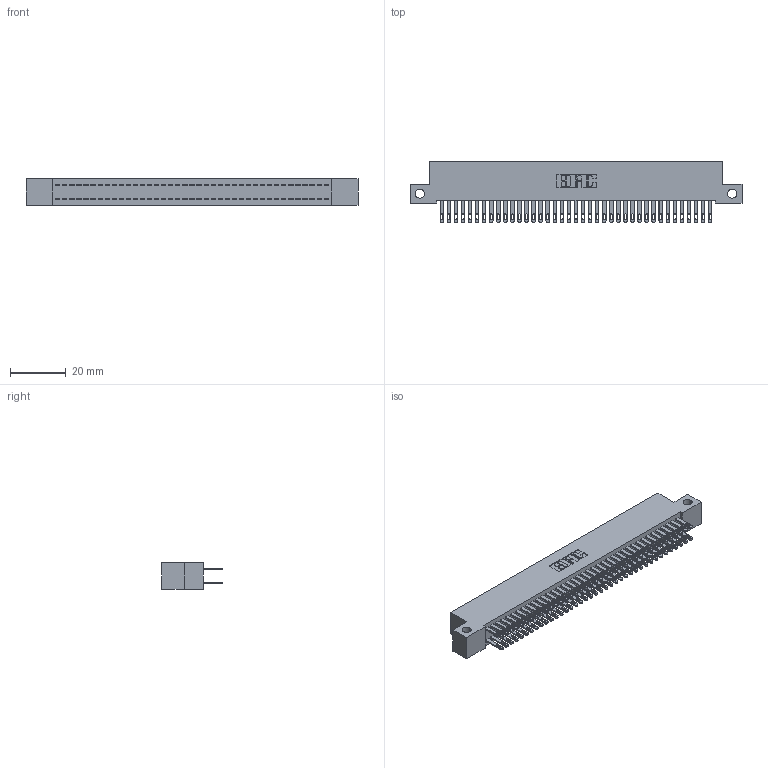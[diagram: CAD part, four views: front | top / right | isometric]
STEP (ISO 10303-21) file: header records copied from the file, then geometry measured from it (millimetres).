
FILE_DESCRIPTION (( 'STEP AP203' ), '1' );
FILE_NAME ('342-078-500-212.STEP', '2018-08-13T13:03:05', ( '' ), ( '' ), 'SwSTEP 2.0', 'SolidWorks 2016', '' );
FILE_SCHEMA (( 'CONFIG_CONTROL_DESIGN' ));
Length unit declared in the file: inch
Products named in the file (3): 342 Part_Side Mount; 345-292-001_345-293-100; 342-078-500-212
Assembly tree (79 placements, depth 2):
  342-078-500-212
    342 Part_Side Mount
    345-292-001_345-293-100  x78
Bounding box: 119.38 x 21.85 x 9.4 mm (x, y, z)
Volume: 10876.5 mm3; surface area: 18217.3 mm2
Topology: 79 solids, 79 shells, 3854 faces, 11765 edges, 7842 vertices
Faces by surface type: plane 2406, cylinder 1448
Entity records: 25279 total; most frequent: CARTESIAN_POINT 4190, ORIENTED_EDGE 4126, DIRECTION 3587, EDGE_CURVE 2063, LINE 1931, VECTOR 1931, VERTEX_POINT 1374, AXIS2_PLACEMENT_3D 828
